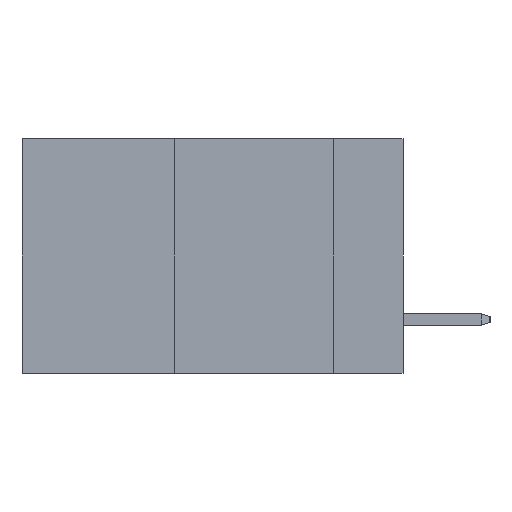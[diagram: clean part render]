
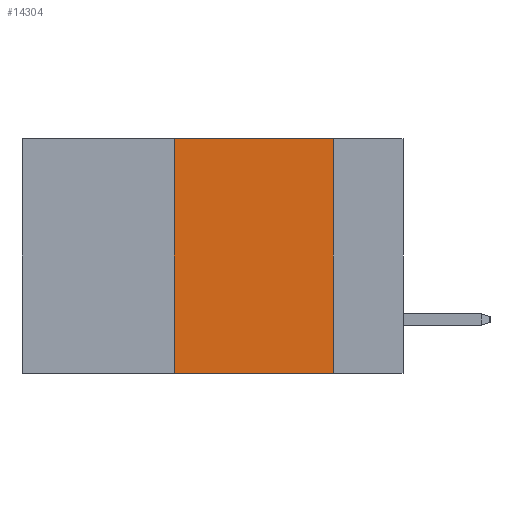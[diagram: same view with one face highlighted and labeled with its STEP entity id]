
A CAD part, left-side view. The second image highlights one B-rep face of the part: STEP entity #14304.
In plain terms, the highlighted planar face has unit normal (-1, 0, 0).
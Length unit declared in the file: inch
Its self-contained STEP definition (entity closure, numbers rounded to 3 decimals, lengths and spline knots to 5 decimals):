
#214 = CARTESIAN_POINT ( 'NONE',  ( 0., 0.6, -0.37 ) ) ;
#409 = CARTESIAN_POINT ( 'NONE',  ( 0., 0.11, 0. ) ) ;
#1020 = LINE ( 'NONE', #8610, #3097 ) ;
#1297 = FACE_OUTER_BOUND ( 'NONE', #8751, .T. ) ;
#1588 = ORIENTED_EDGE ( 'NONE', *, *, #5052, .F. ) ;
#1845 = ORIENTED_EDGE ( 'NONE', *, *, #4061, .F. ) ;
#2111 = ORIENTED_EDGE ( 'NONE', *, *, #14770, .F. ) ;
#2198 = CARTESIAN_POINT ( 'NONE',  ( 0., 0.11, 0. ) ) ;
#3097 = VECTOR ( 'NONE', #8377, 39.37008 ) ;
#3485 = VERTEX_POINT ( 'NONE', #12462 ) ;
#4061 = EDGE_CURVE ( 'NONE', #15201, #3485, #11368, .T. ) ;
#4444 = CARTESIAN_POINT ( 'NONE',  ( 0., 0.36, 0. ) ) ;
#4578 = VERTEX_POINT ( 'NONE', #15267 ) ;
#5014 = LINE ( 'NONE', #214, #7332 ) ;
#5052 = EDGE_CURVE ( 'NONE', #8147, #15201, #1020, .T. ) ;
#6236 = DIRECTION ( 'NONE',  ( 1., 0., 0. ) ) ;
#7332 = VECTOR ( 'NONE', #9895, 39.37008 ) ;
#7934 = DIRECTION ( 'NONE',  ( 0., 0., -1. ) ) ;
#8147 = VERTEX_POINT ( 'NONE', #4444 ) ;
#8377 = DIRECTION ( 'NONE',  ( 0., -1., 0. ) ) ;
#8610 = CARTESIAN_POINT ( 'NONE',  ( 0., 0.6, 0. ) ) ;
#8664 = CARTESIAN_POINT ( 'NONE',  ( 0., 0.6, 0. ) ) ;
#8751 = EDGE_LOOP ( 'NONE', ( #1845, #1588, #2111, #15482 ) ) ;
#9108 = LINE ( 'NONE', #15464, #11169 ) ;
#9895 = DIRECTION ( 'NONE',  ( 0., -1., 0. ) ) ;
#10474 = DIRECTION ( 'NONE',  ( 0., 0., 1. ) ) ;
#11056 = PLANE ( 'NONE',  #11669 ) ;
#11169 = VECTOR ( 'NONE', #10474, 39.37008 ) ;
#11368 = LINE ( 'NONE', #409, #11781 ) ;
#11669 = AXIS2_PLACEMENT_3D ( 'NONE', #8664, #6236, #13512 ) ;
#11781 = VECTOR ( 'NONE', #7934, 39.37008 ) ;
#12462 = CARTESIAN_POINT ( 'NONE',  ( 0., 0.11, -0.37 ) ) ;
#13512 = DIRECTION ( 'NONE',  ( 0., 0., -1. ) ) ;
#14061 = EDGE_CURVE ( 'NONE', #4578, #3485, #5014, .T. ) ;
#14304 = ADVANCED_FACE ( 'NONE', ( #1297 ), #11056, .F. ) ;
#14770 = EDGE_CURVE ( 'NONE', #4578, #8147, #9108, .T. ) ;
#15201 = VERTEX_POINT ( 'NONE', #2198 ) ;
#15267 = CARTESIAN_POINT ( 'NONE',  ( 0., 0.36, -0.37 ) ) ;
#15464 = CARTESIAN_POINT ( 'NONE',  ( 0., 0.36, 0. ) ) ;
#15482 = ORIENTED_EDGE ( 'NONE', *, *, #14061, .T. ) ;
